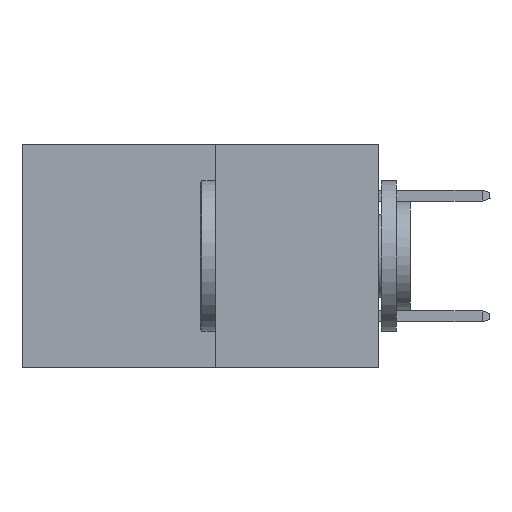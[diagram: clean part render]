
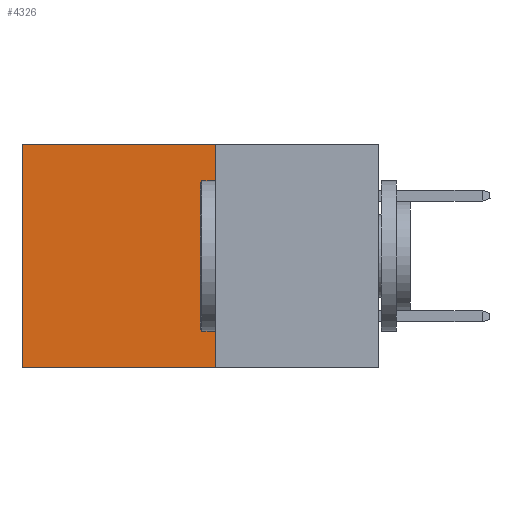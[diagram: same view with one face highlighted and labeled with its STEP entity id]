
A CAD part, left-side view. The second image highlights one B-rep face of the part: STEP entity #4326.
In plain terms, the highlighted planar face has unit normal (-1, 0, 0).
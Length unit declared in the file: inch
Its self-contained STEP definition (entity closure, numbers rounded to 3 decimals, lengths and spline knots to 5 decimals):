
#251 = CARTESIAN_POINT ( 'NONE',  ( 0.277, 0.27, -0.37 ) ) ;
#306 = PLANE ( 'NONE',  #8561 ) ;
#1161 = EDGE_CURVE ( 'NONE', #6927, #4114, #5788, .T. ) ;
#1274 = CARTESIAN_POINT ( 'NONE',  ( 0.277, 0.59, -0.37 ) ) ;
#1362 = ORIENTED_EDGE ( 'NONE', *, *, #7261, .F. ) ;
#1394 = DIRECTION ( 'NONE',  ( 1., 0., 0. ) ) ;
#1785 = VECTOR ( 'NONE', #8114, 39.37008 ) ;
#2470 = ORIENTED_EDGE ( 'NONE', *, *, #1161, .T. ) ;
#4114 = VERTEX_POINT ( 'NONE', #10420 ) ;
#4228 = CARTESIAN_POINT ( 'NONE',  ( 0.277, 0.27, -0.37 ) ) ;
#4326 = ADVANCED_FACE ( 'NONE', ( #5997 ), #306, .F. ) ;
#5075 = DIRECTION ( 'NONE',  ( 0., 0., -1. ) ) ;
#5788 = LINE ( 'NONE', #15744, #8660 ) ;
#5997 = FACE_OUTER_BOUND ( 'NONE', #11569, .T. ) ;
#6289 = DIRECTION ( 'NONE',  ( 0., 1., 0. ) ) ;
#6423 = CARTESIAN_POINT ( 'NONE',  ( 0.277, 0.27, -0.37 ) ) ;
#6881 = CARTESIAN_POINT ( 'NONE',  ( 0.277, 0.59, -0.37 ) ) ;
#6927 = VERTEX_POINT ( 'NONE', #12756 ) ;
#7084 = ORIENTED_EDGE ( 'NONE', *, *, #9860, .T. ) ;
#7229 = DIRECTION ( 'NONE',  ( 0., 0., -1. ) ) ;
#7261 = EDGE_CURVE ( 'NONE', #8542, #14147, #9583, .T. ) ;
#7508 = VECTOR ( 'NONE', #7229, 39.37008 ) ;
#8114 = DIRECTION ( 'NONE',  ( 0., 0., -1. ) ) ;
#8284 = LINE ( 'NONE', #6881, #1785 ) ;
#8542 = VERTEX_POINT ( 'NONE', #4228 ) ;
#8561 = AXIS2_PLACEMENT_3D ( 'NONE', #251, #1394, #5075 ) ;
#8660 = VECTOR ( 'NONE', #14105, 39.37008 ) ;
#9583 = LINE ( 'NONE', #6423, #15673 ) ;
#9860 = EDGE_CURVE ( 'NONE', #4114, #14147, #8284, .T. ) ;
#10420 = CARTESIAN_POINT ( 'NONE',  ( 0.277, 0.59, 0. ) ) ;
#10693 = EDGE_CURVE ( 'NONE', #6927, #8542, #11956, .T. ) ;
#11548 = ORIENTED_EDGE ( 'NONE', *, *, #10693, .F. ) ;
#11569 = EDGE_LOOP ( 'NONE', ( #7084, #1362, #11548, #2470 ) ) ;
#11956 = LINE ( 'NONE', #15709, #7508 ) ;
#12756 = CARTESIAN_POINT ( 'NONE',  ( 0.277, 0.27, 0. ) ) ;
#14105 = DIRECTION ( 'NONE',  ( 0., 1., 0. ) ) ;
#14147 = VERTEX_POINT ( 'NONE', #1274 ) ;
#15673 = VECTOR ( 'NONE', #6289, 39.37008 ) ;
#15709 = CARTESIAN_POINT ( 'NONE',  ( 0.277, 0.27, -0.37 ) ) ;
#15744 = CARTESIAN_POINT ( 'NONE',  ( 0.277, 0.27, 0. ) ) ;
